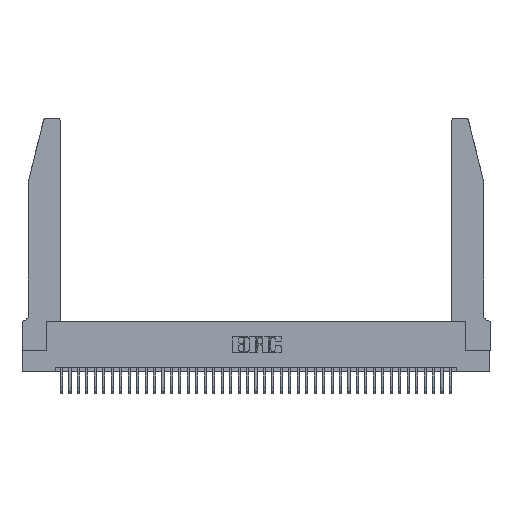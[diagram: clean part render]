
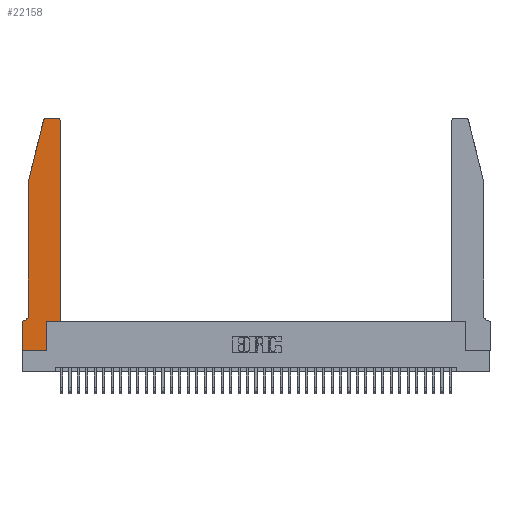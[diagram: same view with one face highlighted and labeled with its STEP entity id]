
A CAD part, top view. The second image highlights one B-rep face of the part: STEP entity #22158.
In plain terms, the highlighted planar face has unit normal (0, 0, 1).
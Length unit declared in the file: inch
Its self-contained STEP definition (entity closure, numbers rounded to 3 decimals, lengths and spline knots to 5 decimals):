
#329 = DIRECTION ( 'NONE',  ( 1., 0., 0. ) ) ;
#464 = VERTEX_POINT ( 'NONE', #29030 ) ;
#793 = LINE ( 'NONE', #23994, #34851 ) ;
#1463 = DIRECTION ( 'NONE',  ( 1., 0., 0. ) ) ;
#1577 = VERTEX_POINT ( 'NONE', #31049 ) ;
#2622 = LINE ( 'NONE', #35170, #36654 ) ;
#3310 = VECTOR ( 'NONE', #13334, 39.37008 ) ;
#3811 = VECTOR ( 'NONE', #27497, 39.37008 ) ;
#4227 = LINE ( 'NONE', #21658, #12031 ) ;
#4338 = CARTESIAN_POINT ( 'NONE',  ( 0.4505, 0.35, 0.37 ) ) ;
#5010 = VERTEX_POINT ( 'NONE', #26078 ) ;
#6513 = EDGE_CURVE ( 'NONE', #19041, #41760, #20959, .T. ) ;
#6665 = CARTESIAN_POINT ( 'NONE',  ( 0.4505, 0.35, 0.37 ) ) ;
#6968 = LINE ( 'NONE', #10473, #23527 ) ;
#7943 = CARTESIAN_POINT ( 'NONE',  ( 0.4205, 2.72, 0.37 ) ) ;
#10196 = ORIENTED_EDGE ( 'NONE', *, *, #42507, .T. ) ;
#10473 = CARTESIAN_POINT ( 'NONE',  ( 0., 0., 0.37 ) ) ;
#11276 = DIRECTION ( 'NONE',  ( 1., 0., 0. ) ) ;
#11351 = CARTESIAN_POINT ( 'NONE',  ( 0., 0.35, 0.37 ) ) ;
#11457 = ORIENTED_EDGE ( 'NONE', *, *, #34097, .T. ) ;
#11474 = ORIENTED_EDGE ( 'NONE', *, *, #40191, .T. ) ;
#11530 = EDGE_CURVE ( 'NONE', #5010, #27051, #31873, .T. ) ;
#11593 = ORIENTED_EDGE ( 'NONE', *, *, #32983, .T. ) ;
#11617 = LINE ( 'NONE', #4338, #3811 ) ;
#12031 = VECTOR ( 'NONE', #37951, 39.37008 ) ;
#12175 = DIRECTION ( 'NONE',  ( 0., -1., 0. ) ) ;
#13334 = DIRECTION ( 'NONE',  ( 0., 1., 0. ) ) ;
#13603 = DIRECTION ( 'NONE',  ( -0.239, -0.971, 0. ) ) ;
#13705 = ORIENTED_EDGE ( 'NONE', *, *, #24448, .T. ) ;
#14457 = CARTESIAN_POINT ( 'NONE',  ( 0., 0., 0.37 ) ) ;
#15359 = DIRECTION ( 'NONE',  ( 0., 0., -1. ) ) ;
#15898 = EDGE_CURVE ( 'NONE', #464, #35427, #4227, .T. ) ;
#15997 = AXIS2_PLACEMENT_3D ( 'NONE', #7943, #31006, #11276 ) ;
#16370 = AXIS2_PLACEMENT_3D ( 'NONE', #34995, #15359, #38259 ) ;
#16862 = FACE_OUTER_BOUND ( 'NONE', #31885, .T. ) ;
#16945 = VERTEX_POINT ( 'NONE', #20438 ) ;
#17015 = LINE ( 'NONE', #37649, #24733 ) ;
#17986 = CARTESIAN_POINT ( 'NONE',  ( 0.25487, 2.72718, 0.37 ) ) ;
#18039 = PLANE ( 'NONE',  #19208 ) ;
#18561 = CIRCLE ( 'NONE', #30273, 0.03 ) ;
#18709 = VECTOR ( 'NONE', #13603, 39.37008 ) ;
#19041 = VERTEX_POINT ( 'NONE', #41225 ) ;
#19208 = AXIS2_PLACEMENT_3D ( 'NONE', #11351, #21336, #1463 ) ;
#19815 = ORIENTED_EDGE ( 'NONE', *, *, #26262, .T. ) ;
#20207 = DIRECTION ( 'NONE',  ( 0., 0., 1. ) ) ;
#20281 = CARTESIAN_POINT ( 'NONE',  ( 0.0755, 2., 0.37 ) ) ;
#20438 = CARTESIAN_POINT ( 'NONE',  ( 0.284, 2.75, 0.37 ) ) ;
#20959 = LINE ( 'NONE', #6665, #3310 ) ;
#21336 = DIRECTION ( 'NONE',  ( 0., 0., 1. ) ) ;
#21346 = DIRECTION ( 'NONE',  ( -1., 0., 0. ) ) ;
#21658 = CARTESIAN_POINT ( 'NONE',  ( 0.2865, 0.35, 0.37 ) ) ;
#22158 = ADVANCED_FACE ( 'NONE', ( #16862 ), #18039, .T. ) ;
#22178 = CARTESIAN_POINT ( 'NONE',  ( 0.0755, 0.42, 0.37 ) ) ;
#22552 = CIRCLE ( 'NONE', #15997, 0.03 ) ;
#23144 = VECTOR ( 'NONE', #40689, 39.37008 ) ;
#23421 = CARTESIAN_POINT ( 'NONE',  ( 0.0755, 2., 0.37 ) ) ;
#23496 = CARTESIAN_POINT ( 'NONE',  ( 0., 0., 0.37 ) ) ;
#23527 = VECTOR ( 'NONE', #26936, 39.37008 ) ;
#23994 = CARTESIAN_POINT ( 'NONE',  ( 0.2605, 2.75, 0.37 ) ) ;
#24322 = CARTESIAN_POINT ( 'NONE',  ( 0.2865, 0.35, 0.37 ) ) ;
#24448 = EDGE_CURVE ( 'NONE', #40294, #32039, #36136, .T. ) ;
#24733 = VECTOR ( 'NONE', #21346, 39.37008 ) ;
#24953 = EDGE_CURVE ( 'NONE', #16945, #40294, #18561, .T. ) ;
#26078 = CARTESIAN_POINT ( 'NONE',  ( 0., 0.35, 0.37 ) ) ;
#26262 = EDGE_CURVE ( 'NONE', #41760, #28017, #22552, .T. ) ;
#26486 = CIRCLE ( 'NONE', #16370, 0.07 ) ;
#26673 = ORIENTED_EDGE ( 'NONE', *, *, #15898, .T. ) ;
#26936 = DIRECTION ( 'NONE',  ( 1., 0., 0. ) ) ;
#27051 = VERTEX_POINT ( 'NONE', #23496 ) ;
#27326 = DIRECTION ( 'NONE',  ( -1., 0., 0. ) ) ;
#27497 = DIRECTION ( 'NONE',  ( 1., 0., 0. ) ) ;
#28017 = VERTEX_POINT ( 'NONE', #41289 ) ;
#29030 = CARTESIAN_POINT ( 'NONE',  ( 0.2865, 0., 0.37 ) ) ;
#29827 = VERTEX_POINT ( 'NONE', #22178 ) ;
#30273 = AXIS2_PLACEMENT_3D ( 'NONE', #39816, #20207, #329 ) ;
#30684 = ORIENTED_EDGE ( 'NONE', *, *, #6513, .T. ) ;
#31006 = DIRECTION ( 'NONE',  ( 0., 0., 1. ) ) ;
#31049 = CARTESIAN_POINT ( 'NONE',  ( 0.0055, 0.35, 0.37 ) ) ;
#31873 = LINE ( 'NONE', #14457, #23144 ) ;
#31885 = EDGE_LOOP ( 'NONE', ( #11457, #36108, #13705, #36915, #10196, #11593, #36170, #34918, #26673, #11474, #30684, #19815 ) ) ;
#32039 = VERTEX_POINT ( 'NONE', #20281 ) ;
#32983 = EDGE_CURVE ( 'NONE', #1577, #5010, #17015, .T. ) ;
#33914 = CARTESIAN_POINT ( 'NONE',  ( 0.4505, 2.72, 0.37 ) ) ;
#34097 = EDGE_CURVE ( 'NONE', #28017, #16945, #793, .T. ) ;
#34851 = VECTOR ( 'NONE', #27326, 39.37008 ) ;
#34918 = ORIENTED_EDGE ( 'NONE', *, *, #40116, .T. ) ;
#34995 = CARTESIAN_POINT ( 'NONE',  ( 0.0055, 0.42, 0.37 ) ) ;
#35170 = CARTESIAN_POINT ( 'NONE',  ( 0.0755, 2., 0.37 ) ) ;
#35427 = VERTEX_POINT ( 'NONE', #24322 ) ;
#36108 = ORIENTED_EDGE ( 'NONE', *, *, #24953, .T. ) ;
#36136 = LINE ( 'NONE', #23421, #18709 ) ;
#36170 = ORIENTED_EDGE ( 'NONE', *, *, #11530, .T. ) ;
#36654 = VECTOR ( 'NONE', #12175, 39.37008 ) ;
#36915 = ORIENTED_EDGE ( 'NONE', *, *, #42023, .T. ) ;
#37649 = CARTESIAN_POINT ( 'NONE',  ( 0.0755, 0.35, 0.37 ) ) ;
#37951 = DIRECTION ( 'NONE',  ( 0., 1., 0. ) ) ;
#38259 = DIRECTION ( 'NONE',  ( -1., 0., 0. ) ) ;
#39816 = CARTESIAN_POINT ( 'NONE',  ( 0.284, 2.72, 0.37 ) ) ;
#40116 = EDGE_CURVE ( 'NONE', #27051, #464, #6968, .T. ) ;
#40191 = EDGE_CURVE ( 'NONE', #35427, #19041, #11617, .T. ) ;
#40294 = VERTEX_POINT ( 'NONE', #17986 ) ;
#40689 = DIRECTION ( 'NONE',  ( 0., -1., 0. ) ) ;
#41225 = CARTESIAN_POINT ( 'NONE',  ( 0.4505, 0.35, 0.37 ) ) ;
#41289 = CARTESIAN_POINT ( 'NONE',  ( 0.4205, 2.75, 0.37 ) ) ;
#41760 = VERTEX_POINT ( 'NONE', #33914 ) ;
#42023 = EDGE_CURVE ( 'NONE', #32039, #29827, #2622, .T. ) ;
#42507 = EDGE_CURVE ( 'NONE', #29827, #1577, #26486, .T. ) ;
